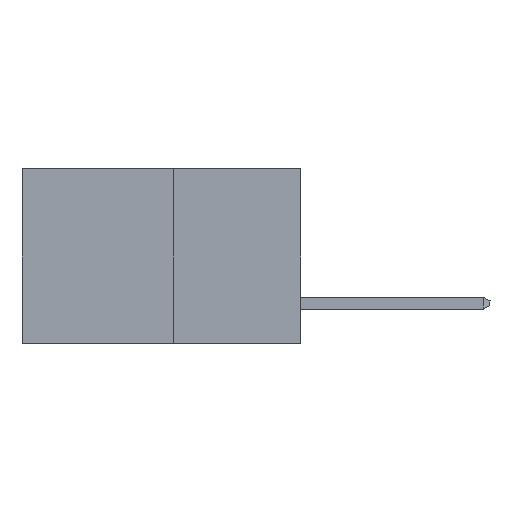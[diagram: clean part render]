
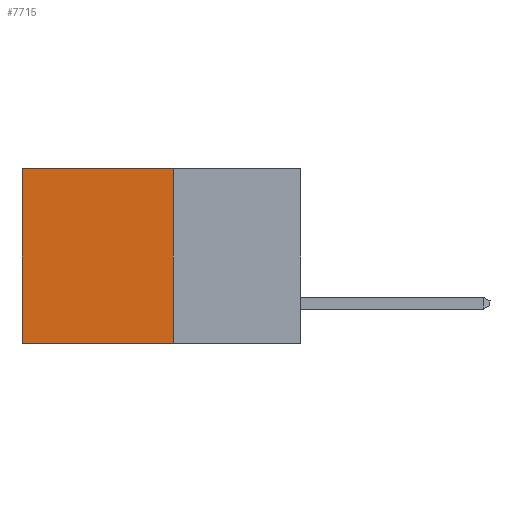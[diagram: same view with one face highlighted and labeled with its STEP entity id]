
A CAD part, left-side view. The second image highlights one B-rep face of the part: STEP entity #7715.
In plain terms, the highlighted planar face has unit normal (-1, 0, 0).
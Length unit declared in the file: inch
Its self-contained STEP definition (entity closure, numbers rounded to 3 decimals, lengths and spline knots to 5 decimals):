
#631 = ORIENTED_EDGE ( 'NONE', *, *, #27278, .T. ) ;
#1516 = CARTESIAN_POINT ( 'NONE',  ( 0.277, 0.27, -0.37 ) ) ;
#1790 = CARTESIAN_POINT ( 'NONE',  ( 0.277, 0.59, 0. ) ) ;
#1809 = EDGE_CURVE ( 'NONE', #7830, #5373, #7522, .T. ) ;
#2151 = DIRECTION ( 'NONE',  ( 0., 0., -1. ) ) ;
#2363 = DIRECTION ( 'NONE',  ( 0., 0., -1. ) ) ;
#4117 = DIRECTION ( 'NONE',  ( 0., 0., -1. ) ) ;
#4912 = CARTESIAN_POINT ( 'NONE',  ( 0.277, 0.27, 0. ) ) ;
#5373 = VERTEX_POINT ( 'NONE', #1516 ) ;
#5772 = CARTESIAN_POINT ( 'NONE',  ( 0.277, 0.27, -0.37 ) ) ;
#6203 = CARTESIAN_POINT ( 'NONE',  ( 0.277, 0.27, 0. ) ) ;
#6895 = EDGE_CURVE ( 'NONE', #12590, #19929, #7740, .T. ) ;
#7522 = LINE ( 'NONE', #5772, #23329 ) ;
#7715 = ADVANCED_FACE ( 'NONE', ( #20214 ), #25879, .F. ) ;
#7740 = LINE ( 'NONE', #23476, #24200 ) ;
#7830 = VERTEX_POINT ( 'NONE', #4912 ) ;
#8031 = ORIENTED_EDGE ( 'NONE', *, *, #1809, .F. ) ;
#9394 = ORIENTED_EDGE ( 'NONE', *, *, #17394, .F. ) ;
#9803 = ORIENTED_EDGE ( 'NONE', *, *, #6895, .T. ) ;
#10482 = DIRECTION ( 'NONE',  ( 0., 1., 0. ) ) ;
#11542 = DIRECTION ( 'NONE',  ( 0., 1., 0. ) ) ;
#12590 = VERTEX_POINT ( 'NONE', #1790 ) ;
#13117 = CARTESIAN_POINT ( 'NONE',  ( 0.277, 0.27, -0.37 ) ) ;
#14593 = EDGE_LOOP ( 'NONE', ( #9803, #9394, #8031, #631 ) ) ;
#15291 = DIRECTION ( 'NONE',  ( 1., 0., 0. ) ) ;
#15632 = VECTOR ( 'NONE', #11542, 39.37008 ) ;
#17005 = LINE ( 'NONE', #18025, #15632 ) ;
#17394 = EDGE_CURVE ( 'NONE', #5373, #19929, #17005, .T. ) ;
#18025 = CARTESIAN_POINT ( 'NONE',  ( 0.277, 0.27, -0.37 ) ) ;
#18800 = VECTOR ( 'NONE', #10482, 39.37008 ) ;
#19929 = VERTEX_POINT ( 'NONE', #22901 ) ;
#20214 = FACE_OUTER_BOUND ( 'NONE', #14593, .T. ) ;
#22901 = CARTESIAN_POINT ( 'NONE',  ( 0.277, 0.59, -0.37 ) ) ;
#23329 = VECTOR ( 'NONE', #2151, 39.37008 ) ;
#23476 = CARTESIAN_POINT ( 'NONE',  ( 0.277, 0.59, -0.37 ) ) ;
#24200 = VECTOR ( 'NONE', #4117, 39.37008 ) ;
#24481 = LINE ( 'NONE', #6203, #18800 ) ;
#25879 = PLANE ( 'NONE',  #27217 ) ;
#27217 = AXIS2_PLACEMENT_3D ( 'NONE', #13117, #15291, #2363 ) ;
#27278 = EDGE_CURVE ( 'NONE', #7830, #12590, #24481, .T. ) ;
